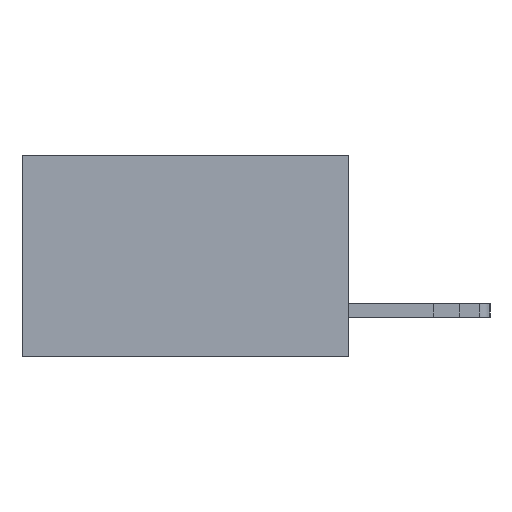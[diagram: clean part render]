
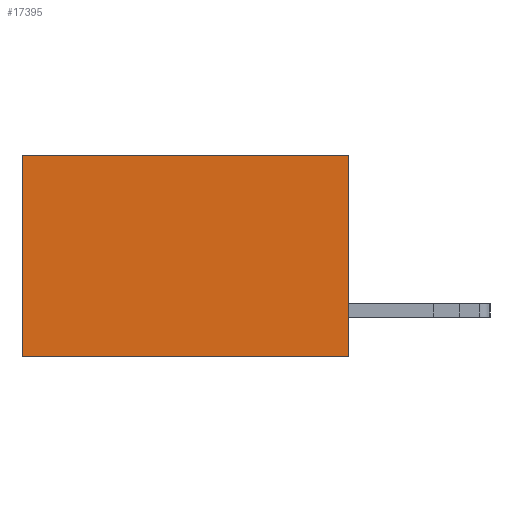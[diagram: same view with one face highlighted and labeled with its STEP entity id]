
A CAD part, left-side view. The second image highlights one B-rep face of the part: STEP entity #17395.
In plain terms, the highlighted planar face has unit normal (-1, 0, 0).
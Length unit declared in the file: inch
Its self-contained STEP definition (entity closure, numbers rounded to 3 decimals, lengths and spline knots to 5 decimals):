
#326 = ORIENTED_EDGE ( 'NONE', *, *, #19066, .T. ) ;
#1181 = CARTESIAN_POINT ( 'NONE',  ( 0.2615, 0.6, 0. ) ) ;
#1230 = LINE ( 'NONE', #6056, #5999 ) ;
#1313 = EDGE_CURVE ( 'NONE', #19564, #16179, #9345, .T. ) ;
#1654 = ORIENTED_EDGE ( 'NONE', *, *, #1313, .F. ) ;
#2348 = ORIENTED_EDGE ( 'NONE', *, *, #20192, .T. ) ;
#3524 = LINE ( 'NONE', #10904, #19473 ) ;
#3650 = VERTEX_POINT ( 'NONE', #7836 ) ;
#5041 = VECTOR ( 'NONE', #12743, 39.37008 ) ;
#5410 = LINE ( 'NONE', #7472, #9219 ) ;
#5638 = AXIS2_PLACEMENT_3D ( 'NONE', #8145, #19221, #9788 ) ;
#5999 = VECTOR ( 'NONE', #18817, 39.37008 ) ;
#6056 = CARTESIAN_POINT ( 'NONE',  ( 0.2615, 0., 0. ) ) ;
#7472 = CARTESIAN_POINT ( 'NONE',  ( 0.2615, 0., -0.37 ) ) ;
#7836 = CARTESIAN_POINT ( 'NONE',  ( 0.2615, 0., 0. ) ) ;
#8145 = CARTESIAN_POINT ( 'NONE',  ( 0.2615, 0., -0.37 ) ) ;
#9219 = VECTOR ( 'NONE', #20138, 39.37008 ) ;
#9345 = LINE ( 'NONE', #12937, #5041 ) ;
#9368 = DIRECTION ( 'NONE',  ( 0., 0., -1. ) ) ;
#9788 = DIRECTION ( 'NONE',  ( 0., 0., -1. ) ) ;
#10904 = CARTESIAN_POINT ( 'NONE',  ( 0.2615, 0.6, -0.37 ) ) ;
#12566 = CARTESIAN_POINT ( 'NONE',  ( 0.2615, 0.6, -0.37 ) ) ;
#12743 = DIRECTION ( 'NONE',  ( 0., 1., 0. ) ) ;
#12937 = CARTESIAN_POINT ( 'NONE',  ( 0.2615, 0., -0.37 ) ) ;
#13500 = ORIENTED_EDGE ( 'NONE', *, *, #17780, .F. ) ;
#14190 = VERTEX_POINT ( 'NONE', #1181 ) ;
#14470 = PLANE ( 'NONE',  #5638 ) ;
#16179 = VERTEX_POINT ( 'NONE', #12566 ) ;
#16677 = FACE_OUTER_BOUND ( 'NONE', #19548, .T. ) ;
#17395 = ADVANCED_FACE ( 'NONE', ( #16677 ), #14470, .F. ) ;
#17780 = EDGE_CURVE ( 'NONE', #3650, #19564, #5410, .T. ) ;
#18817 = DIRECTION ( 'NONE',  ( 0., 1., 0. ) ) ;
#19066 = EDGE_CURVE ( 'NONE', #14190, #16179, #3524, .T. ) ;
#19221 = DIRECTION ( 'NONE',  ( 1., 0., 0. ) ) ;
#19473 = VECTOR ( 'NONE', #9368, 39.37008 ) ;
#19548 = EDGE_LOOP ( 'NONE', ( #326, #1654, #13500, #2348 ) ) ;
#19564 = VERTEX_POINT ( 'NONE', #20143 ) ;
#20138 = DIRECTION ( 'NONE',  ( 0., 0., -1. ) ) ;
#20143 = CARTESIAN_POINT ( 'NONE',  ( 0.2615, 0., -0.37 ) ) ;
#20192 = EDGE_CURVE ( 'NONE', #3650, #14190, #1230, .T. ) ;
